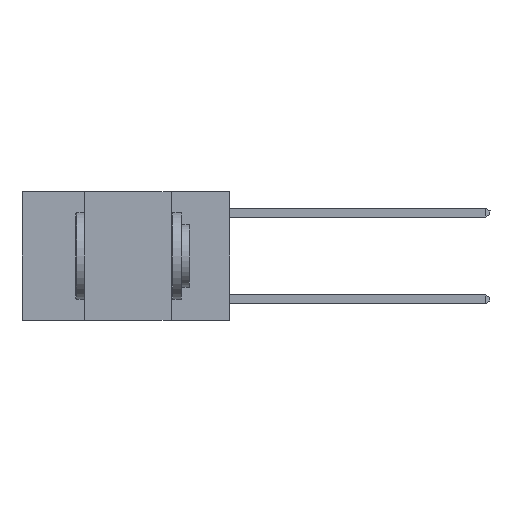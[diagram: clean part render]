
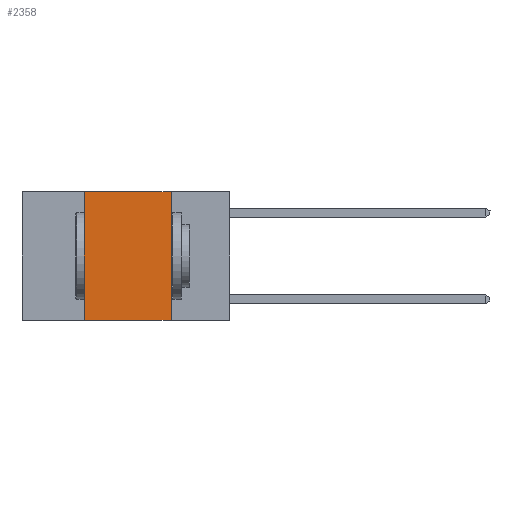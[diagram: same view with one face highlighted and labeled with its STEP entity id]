
A CAD part, left-side view. The second image highlights one B-rep face of the part: STEP entity #2358.
In plain terms, the highlighted planar face has unit normal (-1, 0, 0).
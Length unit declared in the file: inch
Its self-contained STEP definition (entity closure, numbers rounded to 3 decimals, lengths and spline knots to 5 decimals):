
#33 = ORIENTED_EDGE ( 'NONE', *, *, #5929, .T. ) ;
#173 = LINE ( 'NONE', #9109, #9296 ) ;
#564 = CARTESIAN_POINT ( 'NONE',  ( 0., 0.17, 0. ) ) ;
#1787 = ORIENTED_EDGE ( 'NONE', *, *, #5869, .F. ) ;
#2095 = VERTEX_POINT ( 'NONE', #2578 ) ;
#2358 = ADVANCED_FACE ( 'NONE', ( #4737 ), #6268, .F. ) ;
#2520 = DIRECTION ( 'NONE',  ( 1., 0., 0. ) ) ;
#2578 = CARTESIAN_POINT ( 'NONE',  ( 0., 0.17, 0. ) ) ;
#2610 = CARTESIAN_POINT ( 'NONE',  ( 0., 0.6, 0. ) ) ;
#2697 = VERTEX_POINT ( 'NONE', #3976 ) ;
#2796 = AXIS2_PLACEMENT_3D ( 'NONE', #2610, #2520, #8516 ) ;
#3200 = EDGE_CURVE ( 'NONE', #2697, #2095, #7303, .T. ) ;
#3704 = DIRECTION ( 'NONE',  ( 0., 0., 1. ) ) ;
#3976 = CARTESIAN_POINT ( 'NONE',  ( 0., 0.42, 0. ) ) ;
#4166 = DIRECTION ( 'NONE',  ( 0., 0., -1. ) ) ;
#4308 = ORIENTED_EDGE ( 'NONE', *, *, #3200, .F. ) ;
#4737 = FACE_OUTER_BOUND ( 'NONE', #9134, .T. ) ;
#5157 = CARTESIAN_POINT ( 'NONE',  ( 0., 0.6, 0. ) ) ;
#5869 = EDGE_CURVE ( 'NONE', #8646, #2697, #8916, .T. ) ;
#5929 = EDGE_CURVE ( 'NONE', #8646, #9051, #173, .T. ) ;
#6107 = EDGE_CURVE ( 'NONE', #2095, #9051, #7156, .T. ) ;
#6268 = PLANE ( 'NONE',  #2796 ) ;
#7043 = VECTOR ( 'NONE', #3704, 39.37008 ) ;
#7156 = LINE ( 'NONE', #564, #8000 ) ;
#7196 = ORIENTED_EDGE ( 'NONE', *, *, #6107, .F. ) ;
#7303 = LINE ( 'NONE', #5157, #8780 ) ;
#7663 = CARTESIAN_POINT ( 'NONE',  ( 0., 0.17, -0.37 ) ) ;
#7812 = CARTESIAN_POINT ( 'NONE',  ( 0., 0.42, -0.37 ) ) ;
#8000 = VECTOR ( 'NONE', #4166, 39.37008 ) ;
#8059 = CARTESIAN_POINT ( 'NONE',  ( 0., 0.42, 0. ) ) ;
#8060 = DIRECTION ( 'NONE',  ( 0., -1., 0. ) ) ;
#8393 = DIRECTION ( 'NONE',  ( 0., -1., 0. ) ) ;
#8516 = DIRECTION ( 'NONE',  ( 0., 0., -1. ) ) ;
#8646 = VERTEX_POINT ( 'NONE', #7812 ) ;
#8780 = VECTOR ( 'NONE', #8060, 39.37008 ) ;
#8916 = LINE ( 'NONE', #8059, #7043 ) ;
#9051 = VERTEX_POINT ( 'NONE', #7663 ) ;
#9109 = CARTESIAN_POINT ( 'NONE',  ( 0., 0.6, -0.37 ) ) ;
#9134 = EDGE_LOOP ( 'NONE', ( #7196, #4308, #1787, #33 ) ) ;
#9296 = VECTOR ( 'NONE', #8393, 39.37008 ) ;
